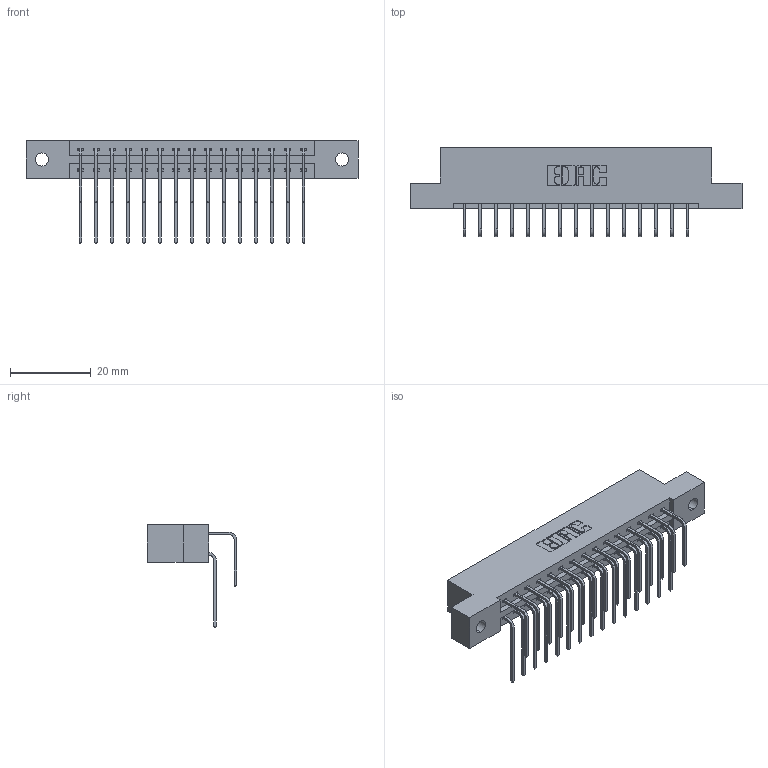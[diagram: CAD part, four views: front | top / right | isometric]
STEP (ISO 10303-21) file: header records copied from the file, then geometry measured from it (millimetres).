
FILE_DESCRIPTION (( 'STEP AP203' ), '1' );
FILE_NAME ('387-030-558-202.STEP', '2019-10-17T15:00:30', ( '' ), ( '' ), 'SwSTEP 2.0', 'SolidWorks 2016', '' );
FILE_SCHEMA (( 'CONFIG_CONTROL_DESIGN' ));
Length unit declared in the file: inch
Products named in the file (4): 387-030-558-202; 337 Part_Flush Mounting Lugs - 0.128 Dia; 345-292-001_558 559 Tail - 1; 345-292-001_558 Tail - 2
Assembly tree (31 placements, depth 2):
  387-030-558-202
    337 Part_Flush Mounting Lugs - 0.128 Dia
    345-292-001_558 559 Tail - 1  x15
    345-292-001_558 Tail - 2  x15
Bounding box: 82.45 x 22.17 x 25.53 mm (x, y, z)
Volume: 8466 mm3; surface area: 9904.9 mm2
Topology: 31 solids, 31 shells, 1794 faces, 5321 edges, 3506 vertices
Faces by surface type: plane 1270, cylinder 524
Entity records: 16909 total; most frequent: CARTESIAN_POINT 2917, ORIENTED_EDGE 2802, DIRECTION 2513, EDGE_CURVE 1401, VECTOR 1233, LINE 1233, VERTEX_POINT 930, AXIS2_PLACEMENT_3D 640
